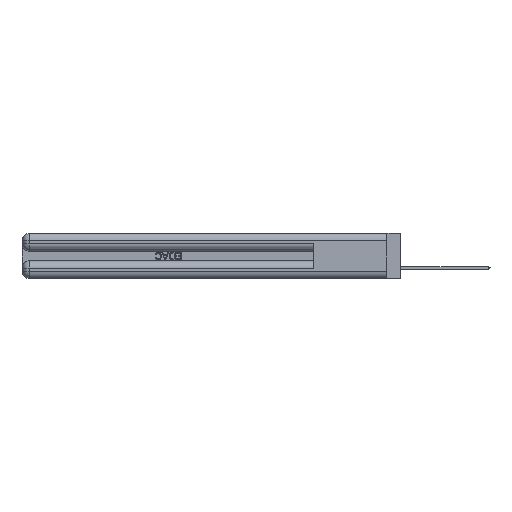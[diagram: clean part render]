
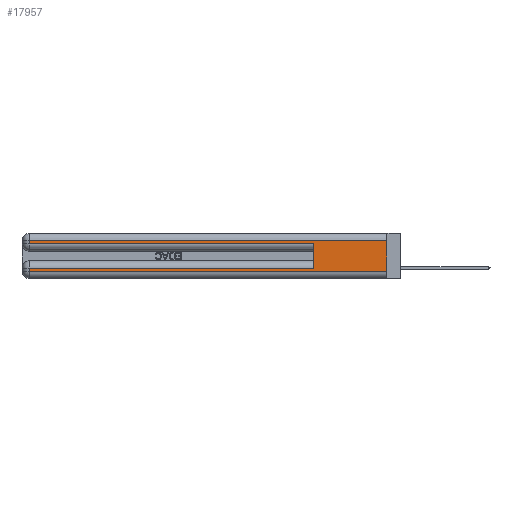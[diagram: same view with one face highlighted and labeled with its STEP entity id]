
A CAD part, left-side view. The second image highlights one B-rep face of the part: STEP entity #17957.
In plain terms, the highlighted planar face has unit normal (-1, 0, 0).
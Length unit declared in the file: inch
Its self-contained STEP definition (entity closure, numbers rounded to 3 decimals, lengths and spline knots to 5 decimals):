
#695 = CARTESIAN_POINT ( 'NONE',  ( 0., 2.94, 0.085 ) ) ;
#2178 = LINE ( 'NONE', #14579, #42142 ) ;
#2598 = FACE_OUTER_BOUND ( 'NONE', #21544, .T. ) ;
#2633 = EDGE_CURVE ( 'NONE', #14144, #34416, #4633, .T. ) ;
#3192 = CARTESIAN_POINT ( 'NONE',  ( 0., 0., 0.31 ) ) ;
#3620 = VECTOR ( 'NONE', #5241, 39.37008 ) ;
#4232 = DIRECTION ( 'NONE',  ( 0., 0., -1. ) ) ;
#4633 = LINE ( 'NONE', #20132, #34991 ) ;
#5241 = DIRECTION ( 'NONE',  ( 0., -1., 0. ) ) ;
#6402 = EDGE_CURVE ( 'NONE', #28830, #28073, #33038, .T. ) ;
#6462 = ORIENTED_EDGE ( 'NONE', *, *, #2633, .T. ) ;
#7853 = PLANE ( 'NONE',  #36778 ) ;
#8564 = VECTOR ( 'NONE', #12405, 39.37008 ) ;
#9793 = CARTESIAN_POINT ( 'NONE',  ( 0., 2.94, 0.31 ) ) ;
#11056 = LINE ( 'NONE', #35938, #3620 ) ;
#12405 = DIRECTION ( 'NONE',  ( 0., 0., -1. ) ) ;
#12556 = CARTESIAN_POINT ( 'NONE',  ( 0., 0.6, 0.145 ) ) ;
#13661 = LINE ( 'NONE', #20588, #16938 ) ;
#14144 = VERTEX_POINT ( 'NONE', #695 ) ;
#14579 = CARTESIAN_POINT ( 'NONE',  ( 0., 0., 0.06 ) ) ;
#15848 = ORIENTED_EDGE ( 'NONE', *, *, #16840, .T. ) ;
#16840 = EDGE_CURVE ( 'NONE', #34416, #19707, #2178, .T. ) ;
#16938 = VECTOR ( 'NONE', #20739, 39.37008 ) ;
#16959 = VECTOR ( 'NONE', #28116, 39.37008 ) ;
#17329 = CARTESIAN_POINT ( 'NONE',  ( 0., 2.94, 0.06 ) ) ;
#17957 = ADVANCED_FACE ( 'NONE', ( #2598 ), #7853, .F. ) ;
#19640 = CARTESIAN_POINT ( 'NONE',  ( 0., 0., 0.085 ) ) ;
#19707 = VERTEX_POINT ( 'NONE', #23197 ) ;
#19715 = ORIENTED_EDGE ( 'NONE', *, *, #31988, .F. ) ;
#20132 = CARTESIAN_POINT ( 'NONE',  ( 0., 2.94, 0.37 ) ) ;
#20588 = CARTESIAN_POINT ( 'NONE',  ( 0., 0., 0.31 ) ) ;
#20636 = ORIENTED_EDGE ( 'NONE', *, *, #6402, .F. ) ;
#20739 = DIRECTION ( 'NONE',  ( 0., 1., 0. ) ) ;
#21544 = EDGE_LOOP ( 'NONE', ( #19715, #35243, #31157, #33519, #20636, #34390, #6462, #15848 ) ) ;
#22090 = CARTESIAN_POINT ( 'NONE',  ( 0., 0.6, 0.085 ) ) ;
#22560 = EDGE_CURVE ( 'NONE', #28357, #26239, #13661, .T. ) ;
#23197 = CARTESIAN_POINT ( 'NONE',  ( 0., 0., 0.06 ) ) ;
#23504 = LINE ( 'NONE', #41315, #16959 ) ;
#26051 = CARTESIAN_POINT ( 'NONE',  ( 0., 0., 0.37 ) ) ;
#26239 = VERTEX_POINT ( 'NONE', #9793 ) ;
#27961 = VECTOR ( 'NONE', #29368, 39.37008 ) ;
#28073 = VERTEX_POINT ( 'NONE', #39410 ) ;
#28116 = DIRECTION ( 'NONE',  ( 0., 0., -1. ) ) ;
#28357 = VERTEX_POINT ( 'NONE', #3192 ) ;
#28830 = VERTEX_POINT ( 'NONE', #22090 ) ;
#29276 = VECTOR ( 'NONE', #43300, 39.37008 ) ;
#29368 = DIRECTION ( 'NONE',  ( 0., 1., 0. ) ) ;
#30151 = EDGE_CURVE ( 'NONE', #28830, #14144, #38261, .T. ) ;
#31157 = ORIENTED_EDGE ( 'NONE', *, *, #43852, .T. ) ;
#31988 = EDGE_CURVE ( 'NONE', #28357, #19707, #40541, .T. ) ;
#33038 = LINE ( 'NONE', #12556, #29276 ) ;
#33519 = ORIENTED_EDGE ( 'NONE', *, *, #44723, .T. ) ;
#34239 = VERTEX_POINT ( 'NONE', #44338 ) ;
#34390 = ORIENTED_EDGE ( 'NONE', *, *, #30151, .T. ) ;
#34416 = VERTEX_POINT ( 'NONE', #17329 ) ;
#34991 = VECTOR ( 'NONE', #4232, 39.37008 ) ;
#35243 = ORIENTED_EDGE ( 'NONE', *, *, #22560, .T. ) ;
#35405 = DIRECTION ( 'NONE',  ( 0., 0., -1. ) ) ;
#35855 = CARTESIAN_POINT ( 'NONE',  ( 0., 0., 0.37 ) ) ;
#35938 = CARTESIAN_POINT ( 'NONE',  ( 0., 0., 0.285 ) ) ;
#36778 = AXIS2_PLACEMENT_3D ( 'NONE', #35855, #42493, #35405 ) ;
#38261 = LINE ( 'NONE', #19640, #27961 ) ;
#38855 = DIRECTION ( 'NONE',  ( 0., -1., 0. ) ) ;
#39410 = CARTESIAN_POINT ( 'NONE',  ( 0., 0.6, 0.285 ) ) ;
#40541 = LINE ( 'NONE', #26051, #8564 ) ;
#41315 = CARTESIAN_POINT ( 'NONE',  ( 0., 2.94, 0.37 ) ) ;
#42142 = VECTOR ( 'NONE', #38855, 39.37008 ) ;
#42493 = DIRECTION ( 'NONE',  ( 1., 0., 0. ) ) ;
#43300 = DIRECTION ( 'NONE',  ( 0., 0., 1. ) ) ;
#43852 = EDGE_CURVE ( 'NONE', #26239, #34239, #23504, .T. ) ;
#44338 = CARTESIAN_POINT ( 'NONE',  ( 0., 2.94, 0.285 ) ) ;
#44723 = EDGE_CURVE ( 'NONE', #34239, #28073, #11056, .T. ) ;
